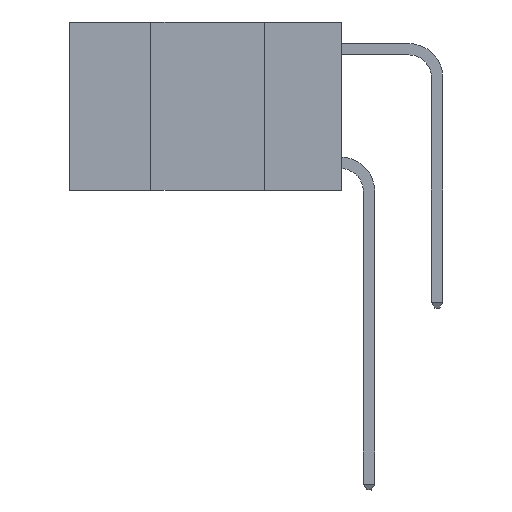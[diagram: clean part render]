
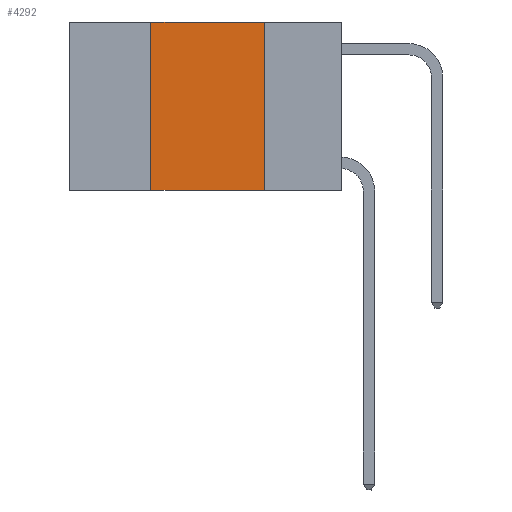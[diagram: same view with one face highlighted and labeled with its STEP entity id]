
A CAD part, left-side view. The second image highlights one B-rep face of the part: STEP entity #4292.
In plain terms, the highlighted planar face has unit normal (-1, 0, 0).
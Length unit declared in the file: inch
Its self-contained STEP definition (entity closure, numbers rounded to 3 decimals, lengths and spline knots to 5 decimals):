
#374 = CARTESIAN_POINT ( 'NONE',  ( 0., 0.42, 0. ) ) ;
#576 = VERTEX_POINT ( 'NONE', #14740 ) ;
#621 = EDGE_CURVE ( 'NONE', #576, #7278, #11107, .T. ) ;
#1103 = CARTESIAN_POINT ( 'NONE',  ( 0., 0.17, -0.37 ) ) ;
#1111 = CARTESIAN_POINT ( 'NONE',  ( 0., 0.6, -0.37 ) ) ;
#2041 = CARTESIAN_POINT ( 'NONE',  ( 0., 0.6, 0. ) ) ;
#2378 = EDGE_CURVE ( 'NONE', #6834, #7278, #9575, .T. ) ;
#2402 = DIRECTION ( 'NONE',  ( 0., -1., 0. ) ) ;
#2890 = ORIENTED_EDGE ( 'NONE', *, *, #3874, .F. ) ;
#3079 = FACE_OUTER_BOUND ( 'NONE', #6081, .T. ) ;
#3166 = AXIS2_PLACEMENT_3D ( 'NONE', #6494, #11442, #12685 ) ;
#3253 = CARTESIAN_POINT ( 'NONE',  ( 0., 0.17, 0. ) ) ;
#3561 = VECTOR ( 'NONE', #2402, 39.37008 ) ;
#3874 = EDGE_CURVE ( 'NONE', #576, #16284, #14942, .T. ) ;
#4157 = ORIENTED_EDGE ( 'NONE', *, *, #13636, .F. ) ;
#4292 = ADVANCED_FACE ( 'NONE', ( #3079 ), #5066, .F. ) ;
#5066 = PLANE ( 'NONE',  #3166 ) ;
#5869 = VECTOR ( 'NONE', #15602, 39.37008 ) ;
#6081 = EDGE_LOOP ( 'NONE', ( #13030, #4157, #2890, #11557 ) ) ;
#6405 = VECTOR ( 'NONE', #14626, 39.37008 ) ;
#6494 = CARTESIAN_POINT ( 'NONE',  ( 0., 0.6, 0. ) ) ;
#6773 = CARTESIAN_POINT ( 'NONE',  ( 0., 0.42, 0. ) ) ;
#6834 = VERTEX_POINT ( 'NONE', #12597 ) ;
#7278 = VERTEX_POINT ( 'NONE', #1103 ) ;
#9575 = LINE ( 'NONE', #3253, #6405 ) ;
#11107 = LINE ( 'NONE', #1111, #3561 ) ;
#11442 = DIRECTION ( 'NONE',  ( 1., 0., 0. ) ) ;
#11557 = ORIENTED_EDGE ( 'NONE', *, *, #621, .T. ) ;
#12597 = CARTESIAN_POINT ( 'NONE',  ( 0., 0.17, 0. ) ) ;
#12685 = DIRECTION ( 'NONE',  ( 0., 0., -1. ) ) ;
#13030 = ORIENTED_EDGE ( 'NONE', *, *, #2378, .F. ) ;
#13179 = VECTOR ( 'NONE', #13300, 39.37008 ) ;
#13300 = DIRECTION ( 'NONE',  ( 0., -1., 0. ) ) ;
#13636 = EDGE_CURVE ( 'NONE', #16284, #6834, #14759, .T. ) ;
#14626 = DIRECTION ( 'NONE',  ( 0., 0., -1. ) ) ;
#14740 = CARTESIAN_POINT ( 'NONE',  ( 0., 0.42, -0.37 ) ) ;
#14759 = LINE ( 'NONE', #2041, #13179 ) ;
#14942 = LINE ( 'NONE', #374, #5869 ) ;
#15602 = DIRECTION ( 'NONE',  ( 0., 0., 1. ) ) ;
#16284 = VERTEX_POINT ( 'NONE', #6773 ) ;
